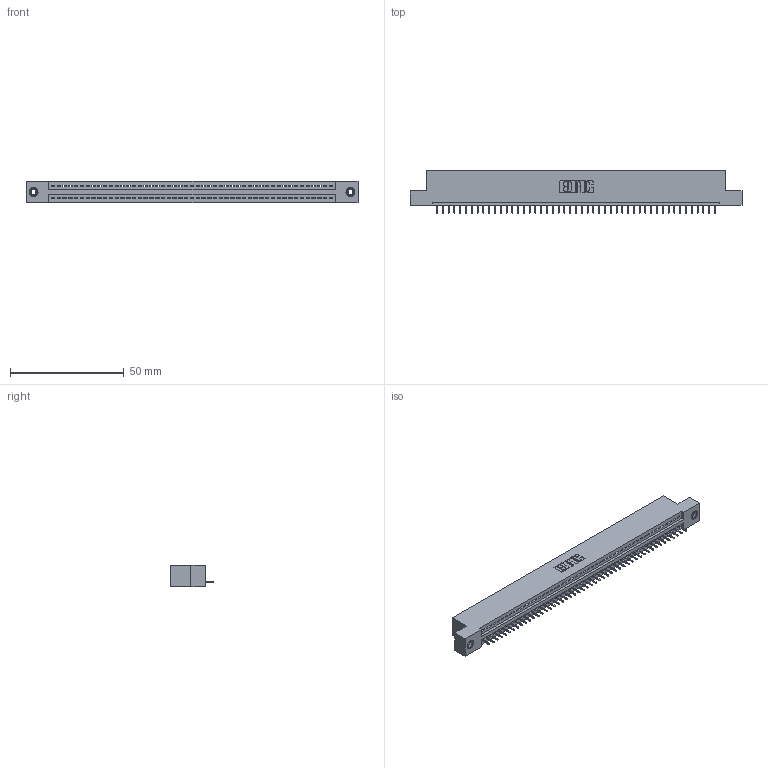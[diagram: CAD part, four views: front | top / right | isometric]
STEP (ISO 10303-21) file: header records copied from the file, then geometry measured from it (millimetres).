
FILE_DESCRIPTION (( 'STEP AP203' ), '1' );
FILE_NAME ('345-049-525-108.STEP', '2020-09-20T01:59:17', ( '' ), ( '' ), 'SwSTEP 2.0', 'SolidWorks 2020', '' );
FILE_SCHEMA (( 'CONFIG_CONTROL_DESIGN' ));
Length unit declared in the file: inch
Products named in the file (4): 345 Part_Flush Mounting Lugs - 0.156 Dia-TI; 345-049-525-108; 345-250-001_345-250-003-102; 345-292-001_345-293-125
Assembly tree (52 placements, depth 2):
  345-049-525-108
    345 Part_Flush Mounting Lugs - 0.156 Dia-TI
    345-292-001_345-293-125  x49
    345-250-001_345-250-003-102  x2
Bounding box: 145.67 x 18.72 x 9.4 mm (x, y, z)
Volume: 13686.6 mm3; surface area: 17635.3 mm2
Topology: 52 solids, 52 shells, 3224 faces, 9297 edges, 5994 vertices
Faces by surface type: plane 2366, cylinder 842, cone 12, torus 4
Entity records: 37196 total; most frequent: CARTESIAN_POINT 6422, ORIENTED_EDGE 6398, DIRECTION 5627, EDGE_CURVE 3199, LINE 2855, VECTOR 2855, VERTEX_POINT 2124, AXIS2_PLACEMENT_3D 1386
